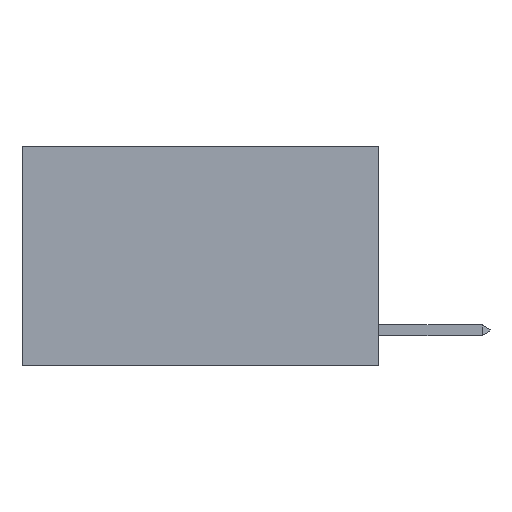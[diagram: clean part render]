
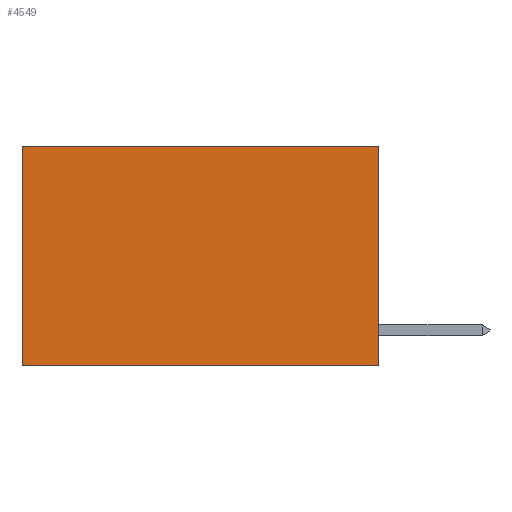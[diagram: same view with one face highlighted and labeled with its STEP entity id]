
A CAD part, left-side view. The second image highlights one B-rep face of the part: STEP entity #4549.
In plain terms, the highlighted planar face has unit normal (-1, 0, 0).
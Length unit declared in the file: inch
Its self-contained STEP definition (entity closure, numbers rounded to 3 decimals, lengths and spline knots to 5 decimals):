
#155 = ORIENTED_EDGE ( 'NONE', *, *, #3556, .F. ) ;
#582 = CARTESIAN_POINT ( 'NONE',  ( 0.2625, 0., -0.37 ) ) ;
#601 = AXIS2_PLACEMENT_3D ( 'NONE', #10022, #7266, #16988 ) ;
#2506 = VECTOR ( 'NONE', #6652, 39.37008 ) ;
#2728 = CARTESIAN_POINT ( 'NONE',  ( 0.2625, 0., -0.37 ) ) ;
#3556 = EDGE_CURVE ( 'NONE', #4160, #7197, #10523, .T. ) ;
#4160 = VERTEX_POINT ( 'NONE', #8666 ) ;
#4549 = ADVANCED_FACE ( 'NONE', ( #12646 ), #5839, .F. ) ;
#4580 = LINE ( 'NONE', #2728, #15294 ) ;
#4653 = EDGE_CURVE ( 'NONE', #13927, #6608, #11323, .T. ) ;
#5608 = ORIENTED_EDGE ( 'NONE', *, *, #4653, .T. ) ;
#5764 = ORIENTED_EDGE ( 'NONE', *, *, #9954, .T. ) ;
#5839 = PLANE ( 'NONE',  #601 ) ;
#6608 = VERTEX_POINT ( 'NONE', #15787 ) ;
#6633 = CARTESIAN_POINT ( 'NONE',  ( 0.2625, 0.6, 0. ) ) ;
#6652 = DIRECTION ( 'NONE',  ( 0., 1., 0. ) ) ;
#7197 = VERTEX_POINT ( 'NONE', #582 ) ;
#7266 = DIRECTION ( 'NONE',  ( 1., 0., 0. ) ) ;
#8044 = VECTOR ( 'NONE', #14399, 39.37008 ) ;
#8666 = CARTESIAN_POINT ( 'NONE',  ( 0.2625, 0., 0. ) ) ;
#8793 = EDGE_CURVE ( 'NONE', #7197, #6608, #4580, .T. ) ;
#8872 = CARTESIAN_POINT ( 'NONE',  ( 0.2625, 0.6, 0. ) ) ;
#9954 = EDGE_CURVE ( 'NONE', #4160, #13927, #9991, .T. ) ;
#9991 = LINE ( 'NONE', #13699, #2506 ) ;
#10022 = CARTESIAN_POINT ( 'NONE',  ( 0.2625, 0., 0. ) ) ;
#10523 = LINE ( 'NONE', #12860, #17880 ) ;
#11172 = DIRECTION ( 'NONE',  ( 0., 1., 0. ) ) ;
#11323 = LINE ( 'NONE', #8872, #8044 ) ;
#12646 = FACE_OUTER_BOUND ( 'NONE', #17784, .T. ) ;
#12860 = CARTESIAN_POINT ( 'NONE',  ( 0.2625, 0., 0. ) ) ;
#13699 = CARTESIAN_POINT ( 'NONE',  ( 0.2625, 0., 0. ) ) ;
#13927 = VERTEX_POINT ( 'NONE', #6633 ) ;
#14399 = DIRECTION ( 'NONE',  ( 0., 0., -1. ) ) ;
#15294 = VECTOR ( 'NONE', #11172, 39.37008 ) ;
#15606 = DIRECTION ( 'NONE',  ( 0., 0., -1. ) ) ;
#15787 = CARTESIAN_POINT ( 'NONE',  ( 0.2625, 0.6, -0.37 ) ) ;
#15935 = ORIENTED_EDGE ( 'NONE', *, *, #8793, .F. ) ;
#16988 = DIRECTION ( 'NONE',  ( 0., 0., -1. ) ) ;
#17784 = EDGE_LOOP ( 'NONE', ( #5608, #15935, #155, #5764 ) ) ;
#17880 = VECTOR ( 'NONE', #15606, 39.37008 ) ;
